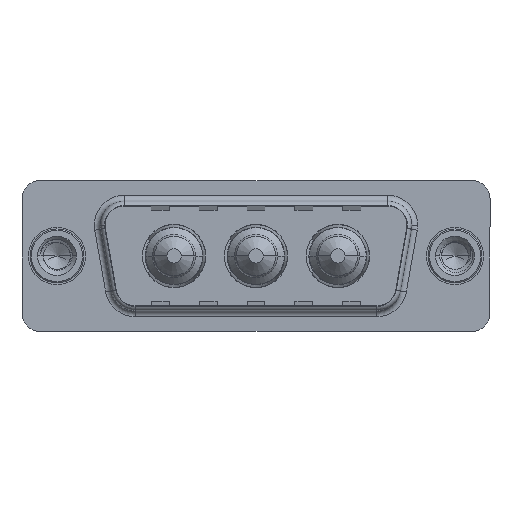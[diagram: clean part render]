
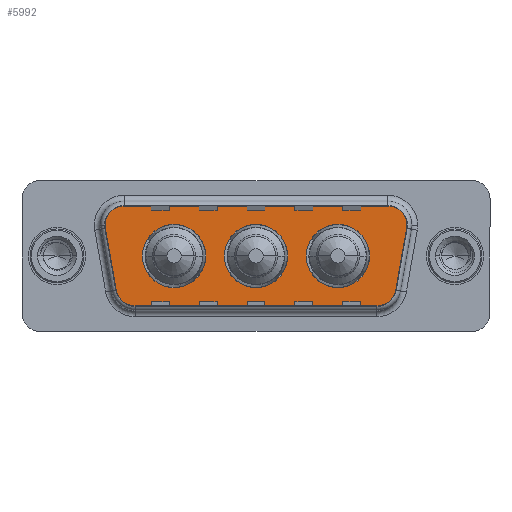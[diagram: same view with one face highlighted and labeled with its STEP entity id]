
A CAD part, top view. The second image highlights one B-rep face of the part: STEP entity #5992.
In plain terms, the highlighted planar face has unit normal (0, 0, 1).
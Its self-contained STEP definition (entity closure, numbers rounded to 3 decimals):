
#229 = EDGE_LOOP ( 'NONE', ( #2416, #5713 ) ) ;
#495 = CARTESIAN_POINT ( 'NONE',  ( 29.859, 2.553, 0. ) ) ;
#520 = CARTESIAN_POINT ( 'NONE',  ( 19.3, 0., 0. ) ) ;
#582 = DIRECTION ( 'NONE',  ( 0., 0., 1. ) ) ;
#897 = VERTEX_POINT ( 'NONE', #12248 ) ;
#1336 = CIRCLE ( 'NONE', #11541, 2. ) ;
#1450 = LINE ( 'NONE', #4009, #11143 ) ;
#1546 = ORIENTED_EDGE ( 'NONE', *, *, #7730, .T. ) ;
#1708 = CARTESIAN_POINT ( 'NONE',  ( 5.411, 2.9, 0. ) ) ;
#1856 = DIRECTION ( 'NONE',  ( 0., 0., 1. ) ) ;
#2025 = CARTESIAN_POINT ( 'NONE',  ( 26.866, -4.9, 0. ) ) ;
#2070 = CARTESIAN_POINT ( 'NONE',  ( 29.859, 2.553, 0. ) ) ;
#2188 = ORIENTED_EDGE ( 'NONE', *, *, #16143, .F. ) ;
#2297 = CIRCLE ( 'NONE', #14261, 2.65 ) ;
#2336 = DIRECTION ( 'NONE',  ( -1., 0., 0. ) ) ;
#2367 = CARTESIAN_POINT ( 'NONE',  ( 6.434, -4.9, 0. ) ) ;
#2416 = ORIENTED_EDGE ( 'NONE', *, *, #3417, .F. ) ;
#2423 = CARTESIAN_POINT ( 'NONE',  ( 16.65, 0., 0. ) ) ;
#2515 = EDGE_CURVE ( 'NONE', #12722, #11615, #9974, .T. ) ;
#2527 = VERTEX_POINT ( 'NONE', #2025 ) ;
#2817 = VERTEX_POINT ( 'NONE', #495 ) ;
#2977 = DIRECTION ( 'NONE',  ( 1., 0., 0. ) ) ;
#3010 = LINE ( 'NONE', #2367, #12660 ) ;
#3029 = AXIS2_PLACEMENT_3D ( 'NONE', #3313, #12140, #4581 ) ;
#3040 = CARTESIAN_POINT ( 'NONE',  ( 26.866, -2.9, 0. ) ) ;
#3215 = VECTOR ( 'NONE', #2336, 1000. ) ;
#3255 = CARTESIAN_POINT ( 'NONE',  ( 20.85, 0., 0. ) ) ;
#3269 = AXIS2_PLACEMENT_3D ( 'NONE', #11722, #4137, #12964 ) ;
#3313 = CARTESIAN_POINT ( 'NONE',  ( 6.434, -2.9, 0. ) ) ;
#3323 = ORIENTED_EDGE ( 'NONE', *, *, #15581, .F. ) ;
#3364 = FACE_BOUND ( 'NONE', #14228, .T. ) ;
#3417 = EDGE_CURVE ( 'NONE', #13025, #6897, #11350, .T. ) ;
#3677 = DIRECTION ( 'NONE',  ( 1., 0., 0. ) ) ;
#4009 = CARTESIAN_POINT ( 'NONE',  ( 3.441, 2.553, 0. ) ) ;
#4116 = VERTEX_POINT ( 'NONE', #4785 ) ;
#4137 = DIRECTION ( 'NONE',  ( 0., 0., 1. ) ) ;
#4292 = DIRECTION ( 'NONE',  ( 1., 0., 0. ) ) ;
#4434 = CARTESIAN_POINT ( 'NONE',  ( 9.8, 0., 0. ) ) ;
#4581 = DIRECTION ( 'NONE',  ( -1., 0., 0. ) ) ;
#4785 = CARTESIAN_POINT ( 'NONE',  ( 7.15, 0., 0. ) ) ;
#4991 = CARTESIAN_POINT ( 'NONE',  ( 27.889, 2.9, 0. ) ) ;
#5085 = ORIENTED_EDGE ( 'NONE', *, *, #10535, .T. ) ;
#5122 = DIRECTION ( 'NONE',  ( 0., 0., 1. ) ) ;
#5263 = AXIS2_PLACEMENT_3D ( 'NONE', #8167, #582, #9456 ) ;
#5560 = CARTESIAN_POINT ( 'NONE',  ( 26.866, -2.9, 0. ) ) ;
#5673 = DIRECTION ( 'NONE',  ( 1., 0., 0. ) ) ;
#5713 = ORIENTED_EDGE ( 'NONE', *, *, #5978, .F. ) ;
#5790 = ORIENTED_EDGE ( 'NONE', *, *, #9284, .F. ) ;
#5978 = EDGE_CURVE ( 'NONE', #6897, #13025, #6319, .T. ) ;
#5992 = ADVANCED_FACE ( 'NONE', ( #3364, #16024, #12624, #9332 ), #15717, .T. ) ;
#6181 = VERTEX_POINT ( 'NONE', #12211 ) ;
#6251 = DIRECTION ( 'NONE',  ( -1., 0., 0. ) ) ;
#6319 = CIRCLE ( 'NONE', #5263, 2.65 ) ;
#6428 = AXIS2_PLACEMENT_3D ( 'NONE', #15273, #5122, #13428 ) ;
#6489 = CARTESIAN_POINT ( 'NONE',  ( 6.434, -4.9, 0. ) ) ;
#6493 = ORIENTED_EDGE ( 'NONE', *, *, #11260, .T. ) ;
#6513 = ORIENTED_EDGE ( 'NONE', *, *, #7034, .F. ) ;
#6518 = VERTEX_POINT ( 'NONE', #14251 ) ;
#6709 = EDGE_LOOP ( 'NONE', ( #7372, #15938, #15934, #1546, #14672, #16228, #7510, #5085, #6493 ) ) ;
#6865 = CIRCLE ( 'NONE', #15605, 2.65 ) ;
#6897 = VERTEX_POINT ( 'NONE', #3255 ) ;
#6975 = CARTESIAN_POINT ( 'NONE',  ( 9.8, 0., 0. ) ) ;
#7034 = EDGE_CURVE ( 'NONE', #6181, #14011, #8540, .T. ) ;
#7170 = CARTESIAN_POINT ( 'NONE',  ( 16.65, 0., 0. ) ) ;
#7372 = ORIENTED_EDGE ( 'NONE', *, *, #14844, .T. ) ;
#7387 = CIRCLE ( 'NONE', #10368, 2. ) ;
#7510 = ORIENTED_EDGE ( 'NONE', *, *, #10840, .T. ) ;
#7730 = EDGE_CURVE ( 'NONE', #8185, #12722, #9500, .T. ) ;
#8167 = CARTESIAN_POINT ( 'NONE',  ( 23.5, 0., 0. ) ) ;
#8185 = VERTEX_POINT ( 'NONE', #10872 ) ;
#8261 = DIRECTION ( 'NONE',  ( 1., 0., 0. ) ) ;
#8459 = DIRECTION ( 'NONE',  ( 1., 0., 0. ) ) ;
#8540 = CIRCLE ( 'NONE', #15347, 2.65 ) ;
#8660 = CIRCLE ( 'NONE', #14820, 2.65 ) ;
#8715 = AXIS2_PLACEMENT_3D ( 'NONE', #5560, #1856, #10731 ) ;
#9284 = EDGE_CURVE ( 'NONE', #4116, #11077, #6865, .T. ) ;
#9332 = FACE_OUTER_BOUND ( 'NONE', #6709, .T. ) ;
#9456 = DIRECTION ( 'NONE',  ( 1., 0., 0. ) ) ;
#9500 = CIRCLE ( 'NONE', #14400, 2. ) ;
#9974 = LINE ( 'NONE', #10944, #3215 ) ;
#10081 = DIRECTION ( 'NONE',  ( 0.174, -0.985, 0. ) ) ;
#10332 = CARTESIAN_POINT ( 'NONE',  ( 26.15, 0., 0. ) ) ;
#10368 = AXIS2_PLACEMENT_3D ( 'NONE', #1708, #10584, #2977 ) ;
#10535 = EDGE_CURVE ( 'NONE', #897, #13016, #14680, .T. ) ;
#10584 = DIRECTION ( 'NONE',  ( 0., 0., 1. ) ) ;
#10730 = CARTESIAN_POINT ( 'NONE',  ( 5.411, 4.9, 0. ) ) ;
#10731 = DIRECTION ( 'NONE',  ( 1., 0., 0. ) ) ;
#10840 = EDGE_CURVE ( 'NONE', #12421, #897, #1450, .T. ) ;
#10872 = CARTESIAN_POINT ( 'NONE',  ( 29.889, 2.9, 0. ) ) ;
#10891 = CARTESIAN_POINT ( 'NONE',  ( 12.45, 0., 0. ) ) ;
#10906 = EDGE_CURVE ( 'NONE', #11615, #12421, #7387, .T. ) ;
#10907 = DIRECTION ( 'NONE',  ( 0.174, 0.985, 0. ) ) ;
#10944 = CARTESIAN_POINT ( 'NONE',  ( 5.411, 4.9, 0. ) ) ;
#11077 = VERTEX_POINT ( 'NONE', #10891 ) ;
#11143 = VECTOR ( 'NONE', #10081, 1000. ) ;
#11165 = EDGE_LOOP ( 'NONE', ( #2188, #5790 ) ) ;
#11190 = VECTOR ( 'NONE', #10907, 1000. ) ;
#11211 = DIRECTION ( 'NONE',  ( 1., 0., 0. ) ) ;
#11260 = EDGE_CURVE ( 'NONE', #13016, #2527, #3010, .T. ) ;
#11267 = DIRECTION ( 'NONE',  ( 0., 0., 1. ) ) ;
#11350 = CIRCLE ( 'NONE', #6428, 2.65 ) ;
#11541 = AXIS2_PLACEMENT_3D ( 'NONE', #3040, #11863, #4292 ) ;
#11615 = VERTEX_POINT ( 'NONE', #10730 ) ;
#11722 = CARTESIAN_POINT ( 'NONE',  ( 27.889, 2.9, 0. ) ) ;
#11863 = DIRECTION ( 'NONE',  ( 0., 0., 1. ) ) ;
#12118 = CARTESIAN_POINT ( 'NONE',  ( 27.889, 4.9, 0. ) ) ;
#12140 = DIRECTION ( 'NONE',  ( 0., 0., 1. ) ) ;
#12211 = CARTESIAN_POINT ( 'NONE',  ( 14., 0., 0. ) ) ;
#12248 = CARTESIAN_POINT ( 'NONE',  ( 4.464, -3.247, 0. ) ) ;
#12421 = VERTEX_POINT ( 'NONE', #14119 ) ;
#12624 = FACE_BOUND ( 'NONE', #11165, .T. ) ;
#12660 = VECTOR ( 'NONE', #11211, 1000. ) ;
#12722 = VERTEX_POINT ( 'NONE', #12118 ) ;
#12964 = DIRECTION ( 'NONE',  ( -1., 0., 0. ) ) ;
#13016 = VERTEX_POINT ( 'NONE', #6489 ) ;
#13025 = VERTEX_POINT ( 'NONE', #10332 ) ;
#13258 = DIRECTION ( 'NONE',  ( 0., 0., 1. ) ) ;
#13428 = DIRECTION ( 'NONE',  ( 1., 0., 0. ) ) ;
#13812 = DIRECTION ( 'NONE',  ( 0., 0., 1. ) ) ;
#14011 = VERTEX_POINT ( 'NONE', #520 ) ;
#14119 = CARTESIAN_POINT ( 'NONE',  ( 3.441, 2.553, 0. ) ) ;
#14228 = EDGE_LOOP ( 'NONE', ( #3323, #6513 ) ) ;
#14251 = CARTESIAN_POINT ( 'NONE',  ( 28.836, -3.247, 0. ) ) ;
#14261 = AXIS2_PLACEMENT_3D ( 'NONE', #6975, #15811, #8261 ) ;
#14330 = CIRCLE ( 'NONE', #3269, 2. ) ;
#14400 = AXIS2_PLACEMENT_3D ( 'NONE', #4991, #13812, #6251 ) ;
#14523 = LINE ( 'NONE', #2070, #11190 ) ;
#14672 = ORIENTED_EDGE ( 'NONE', *, *, #2515, .T. ) ;
#14680 = CIRCLE ( 'NONE', #3029, 2. ) ;
#14820 = AXIS2_PLACEMENT_3D ( 'NONE', #7170, #15998, #8459 ) ;
#14844 = EDGE_CURVE ( 'NONE', #2527, #6518, #1336, .T. ) ;
#15273 = CARTESIAN_POINT ( 'NONE',  ( 23.5, 0., 0. ) ) ;
#15347 = AXIS2_PLACEMENT_3D ( 'NONE', #2423, #11267, #3677 ) ;
#15581 = EDGE_CURVE ( 'NONE', #14011, #6181, #8660, .T. ) ;
#15605 = AXIS2_PLACEMENT_3D ( 'NONE', #4434, #13258, #5673 ) ;
#15717 = PLANE ( 'NONE',  #8715 ) ;
#15811 = DIRECTION ( 'NONE',  ( 0., 0., 1. ) ) ;
#15934 = ORIENTED_EDGE ( 'NONE', *, *, #15986, .T. ) ;
#15938 = ORIENTED_EDGE ( 'NONE', *, *, #16208, .T. ) ;
#15986 = EDGE_CURVE ( 'NONE', #2817, #8185, #14330, .T. ) ;
#15998 = DIRECTION ( 'NONE',  ( 0., 0., 1. ) ) ;
#16024 = FACE_BOUND ( 'NONE', #229, .T. ) ;
#16143 = EDGE_CURVE ( 'NONE', #11077, #4116, #2297, .T. ) ;
#16208 = EDGE_CURVE ( 'NONE', #6518, #2817, #14523, .T. ) ;
#16228 = ORIENTED_EDGE ( 'NONE', *, *, #10906, .T. ) ;
